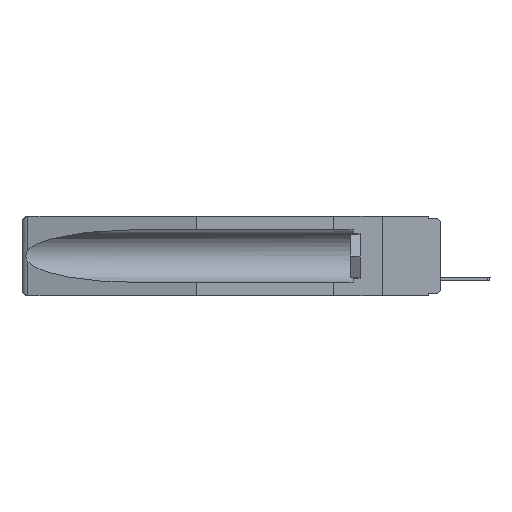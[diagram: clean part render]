
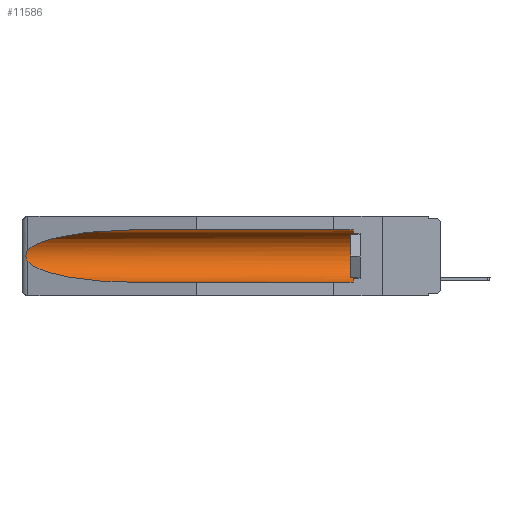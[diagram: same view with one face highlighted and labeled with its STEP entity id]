
A CAD part, left-side view. The second image highlights one B-rep face of the part: STEP entity #11586.
In plain terms, the highlighted cylindrical face has radius 2.857 mm (diameter 5.715 mm), a partial arc.
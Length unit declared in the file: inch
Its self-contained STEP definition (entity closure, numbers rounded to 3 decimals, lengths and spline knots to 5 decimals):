
#702 = VERTEX_POINT ( 'NONE', #9555 ) ;
#1373 = DIRECTION ( 'NONE',  ( 0., 1., 0. ) ) ;
#1533 = EDGE_CURVE ( 'NONE', #10531, #8218, #3028, .T. ) ;
#1901 =( BOUNDED_CURVE ( )  B_SPLINE_CURVE ( 3, ( #8276, #13983, #2329, #4011 ),
 .UNSPECIFIED., .F., .F. ) 
 B_SPLINE_CURVE_WITH_KNOTS ( ( 4, 4 ),
 ( 4.71239, 6.08839 ),
 .UNSPECIFIED. ) 
 CURVE ( )  GEOMETRIC_REPRESENTATION_ITEM ( )  RATIONAL_B_SPLINE_CURVE ( ( 1., 0.848, 0.848, 1. ) ) 
 REPRESENTATION_ITEM ( '' )  );
#2329 = CARTESIAN_POINT ( 'NONE',  ( 0.25451, 1.48313, -0.09465 ) ) ;
#2656 = CIRCLE ( 'NONE', #17383, 0.1125 ) ;
#2956 = ORIENTED_EDGE ( 'NONE', *, *, #14270, .T. ) ;
#3028 = LINE ( 'NONE', #8787, #7900 ) ;
#3135 = CARTESIAN_POINT ( 'NONE',  ( 0.155, -0.30754, -0.059 ) ) ;
#3440 = VECTOR ( 'NONE', #11878, 39.37008 ) ;
#3637 = CARTESIAN_POINT ( 'NONE',  ( 0.25451, 1.48313, -0.24835 ) ) ;
#3669 = EDGE_CURVE ( 'NONE', #9361, #14286, #1901, .T. ) ;
#4011 = CARTESIAN_POINT ( 'NONE',  ( 0.26537, 1.52718, -0.14972 ) ) ;
#4156 = DIRECTION ( 'NONE',  ( 0., 0., 1. ) ) ;
#4209 = FACE_OUTER_BOUND ( 'NONE', #9851, .T. ) ;
#4432 = EDGE_CURVE ( 'NONE', #12777, #9361, #7662, .T. ) ;
#4500 = CARTESIAN_POINT ( 'NONE',  ( 0.26654, 1.53092, -0.15636 ) ) ;
#4849 = CARTESIAN_POINT ( 'NONE',  ( 0.26537, 1.52718, -0.14972 ) ) ;
#5383 = CARTESIAN_POINT ( 'NONE',  ( 0.155, 0.126, -0.1715 ) ) ;
#5737 = CARTESIAN_POINT ( 'NONE',  ( 0.26537, 1.52718, -0.19328 ) ) ;
#6013 = CARTESIAN_POINT ( 'NONE',  ( 0.26655, 1.53094, -0.18657 ) ) ;
#6869 = CARTESIAN_POINT ( 'NONE',  ( 0.155, 0.126, -0.059 ) ) ;
#7436 = CARTESIAN_POINT ( 'NONE',  ( 0.2675, 1.53308, -0.17534 ) ) ;
#7545 = CARTESIAN_POINT ( 'NONE',  ( 0.155, 1.07973, -0.284 ) ) ;
#7662 = LINE ( 'NONE', #3135, #3440 ) ;
#7891 = CARTESIAN_POINT ( 'NONE',  ( 0.21114, 1.30732, -0.284 ) ) ;
#7900 = VECTOR ( 'NONE', #13086, 39.37008 ) ;
#8196 =( BOUNDED_CURVE ( )  B_SPLINE_CURVE ( 3, ( #17754, #3637, #7891, #14923 ),
 .UNSPECIFIED., .F., .F. ) 
 B_SPLINE_CURVE_WITH_KNOTS ( ( 4, 4 ),
 ( 0.1948, 1.5708 ),
 .UNSPECIFIED. ) 
 CURVE ( )  GEOMETRIC_REPRESENTATION_ITEM ( )  RATIONAL_B_SPLINE_CURVE ( ( 1., 0.848, 0.848, 1. ) ) 
 REPRESENTATION_ITEM ( '' )  );
#8218 = VERTEX_POINT ( 'NONE', #7545 ) ;
#8276 = CARTESIAN_POINT ( 'NONE',  ( 0.155, 1.07973, -0.059 ) ) ;
#8443 = EDGE_CURVE ( 'NONE', #14286, #702, #15689, .T. ) ;
#8483 = CARTESIAN_POINT ( 'NONE',  ( 0.2675, 1.53308, -0.16763 ) ) ;
#8787 = CARTESIAN_POINT ( 'NONE',  ( 0.155, -0.30754, -0.284 ) ) ;
#9110 = ORIENTED_EDGE ( 'NONE', *, *, #9127, .T. ) ;
#9127 = EDGE_CURVE ( 'NONE', #10531, #12777, #2656, .T. ) ;
#9361 = VERTEX_POINT ( 'NONE', #15827 ) ;
#9447 = ORIENTED_EDGE ( 'NONE', *, *, #8443, .T. ) ;
#9555 = CARTESIAN_POINT ( 'NONE',  ( 0.26537, 1.52718, -0.19328 ) ) ;
#9851 = EDGE_LOOP ( 'NONE', ( #12871, #9447, #2956, #11714, #9110, #11133 ) ) ;
#9969 = CARTESIAN_POINT ( 'NONE',  ( 0.26597, 1.5296, -0.19026 ) ) ;
#10531 = VERTEX_POINT ( 'NONE', #10857 ) ;
#10857 = CARTESIAN_POINT ( 'NONE',  ( 0.155, 0.126, -0.284 ) ) ;
#11133 = ORIENTED_EDGE ( 'NONE', *, *, #4432, .T. ) ;
#11586 = ADVANCED_FACE ( 'NONE', ( #4209 ), #16051, .F. ) ;
#11714 = ORIENTED_EDGE ( 'NONE', *, *, #1533, .F. ) ;
#11878 = DIRECTION ( 'NONE',  ( 0., 1., 0. ) ) ;
#12777 = VERTEX_POINT ( 'NONE', #6869 ) ;
#12871 = ORIENTED_EDGE ( 'NONE', *, *, #3669, .T. ) ;
#13086 = DIRECTION ( 'NONE',  ( 0., 1., 0. ) ) ;
#13141 = CARTESIAN_POINT ( 'NONE',  ( 0.2673, 1.53269, -0.17917 ) ) ;
#13983 = CARTESIAN_POINT ( 'NONE',  ( 0.21114, 1.30732, -0.059 ) ) ;
#14270 = EDGE_CURVE ( 'NONE', #702, #8218, #8196, .T. ) ;
#14286 = VERTEX_POINT ( 'NONE', #4849 ) ;
#14369 = CARTESIAN_POINT ( 'NONE',  ( 0.155, -0.30754, -0.1715 ) ) ;
#14442 = AXIS2_PLACEMENT_3D ( 'NONE', #14369, #1373, #17290 ) ;
#14923 = CARTESIAN_POINT ( 'NONE',  ( 0.155, 1.07973, -0.284 ) ) ;
#15689 = B_SPLINE_CURVE_WITH_KNOTS ( 'NONE', 3,
 ( #17399, #17480, #4500, #18621, #8483, #7436, #13141, #6013, #9969, #5737 ),
 .UNSPECIFIED., .F., .F.,
 ( 4, 2, 2, 2, 4 ),
 ( 0., 0.00029, 0.00058, 0.00087, 0.00117 ),
 .UNSPECIFIED. ) ;
#15827 = CARTESIAN_POINT ( 'NONE',  ( 0.155, 1.07973, -0.059 ) ) ;
#16051 = CYLINDRICAL_SURFACE ( 'NONE', #14442, 0.1125 ) ;
#17053 = DIRECTION ( 'NONE',  ( 0., -1., 0. ) ) ;
#17290 = DIRECTION ( 'NONE',  ( 0., 0., 1. ) ) ;
#17383 = AXIS2_PLACEMENT_3D ( 'NONE', #5383, #17053, #4156 ) ;
#17399 = CARTESIAN_POINT ( 'NONE',  ( 0.26537, 1.52718, -0.14972 ) ) ;
#17480 = CARTESIAN_POINT ( 'NONE',  ( 0.26597, 1.52961, -0.15275 ) ) ;
#17754 = CARTESIAN_POINT ( 'NONE',  ( 0.26537, 1.52718, -0.19328 ) ) ;
#18621 = CARTESIAN_POINT ( 'NONE',  ( 0.2673, 1.5327, -0.16383 ) ) ;
